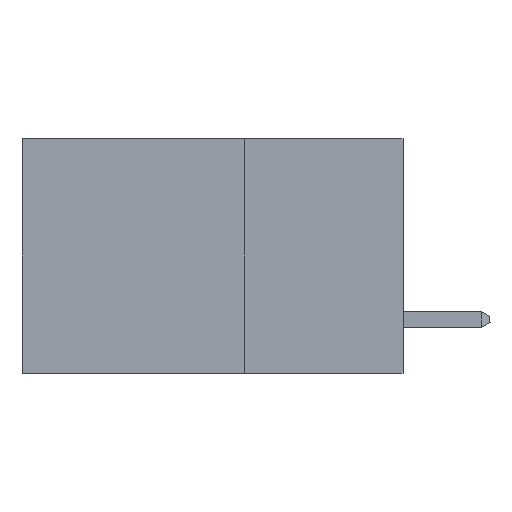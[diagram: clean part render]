
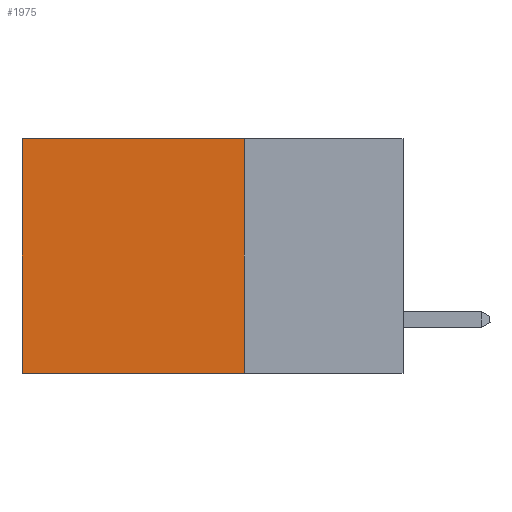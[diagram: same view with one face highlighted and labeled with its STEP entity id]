
A CAD part, left-side view. The second image highlights one B-rep face of the part: STEP entity #1975.
In plain terms, the highlighted planar face has unit normal (-1, 0, 0).
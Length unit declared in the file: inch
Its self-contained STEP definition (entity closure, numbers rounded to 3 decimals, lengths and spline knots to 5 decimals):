
#53 = FACE_OUTER_BOUND ( 'NONE', #13181, .T. ) ;
#1191 = CARTESIAN_POINT ( 'NONE',  ( 0.2875, 0.25, -0.37 ) ) ;
#1975 = ADVANCED_FACE ( 'NONE', ( #53 ), #24681, .F. ) ;
#2242 = ORIENTED_EDGE ( 'NONE', *, *, #23181, .T. ) ;
#3297 = VERTEX_POINT ( 'NONE', #16353 ) ;
#3943 = EDGE_CURVE ( 'NONE', #3297, #7754, #12428, .T. ) ;
#4114 = CARTESIAN_POINT ( 'NONE',  ( 0.2875, 0.6, 0. ) ) ;
#5300 = VECTOR ( 'NONE', #10237, 39.37008 ) ;
#5511 = DIRECTION ( 'NONE',  ( 0., 1., 0. ) ) ;
#7107 = DIRECTION ( 'NONE',  ( 1., 0., 0. ) ) ;
#7754 = VERTEX_POINT ( 'NONE', #9951 ) ;
#7958 = CARTESIAN_POINT ( 'NONE',  ( 0.2875, 0.6, 0. ) ) ;
#8385 = DIRECTION ( 'NONE',  ( 0., 0., -1. ) ) ;
#8970 = ORIENTED_EDGE ( 'NONE', *, *, #15194, .F. ) ;
#9731 = CARTESIAN_POINT ( 'NONE',  ( 0.2875, 0.6, -0.37 ) ) ;
#9815 = LINE ( 'NONE', #16676, #5300 ) ;
#9951 = CARTESIAN_POINT ( 'NONE',  ( 0.2875, 0.25, -0.37 ) ) ;
#10237 = DIRECTION ( 'NONE',  ( 0., 1., 0. ) ) ;
#12428 = LINE ( 'NONE', #23853, #12786 ) ;
#12786 = VECTOR ( 'NONE', #8385, 39.37008 ) ;
#13181 = EDGE_LOOP ( 'NONE', ( #22997, #8970, #25970, #2242 ) ) ;
#15120 = EDGE_CURVE ( 'NONE', #16158, #26685, #21696, .T. ) ;
#15194 = EDGE_CURVE ( 'NONE', #7754, #26685, #18224, .T. ) ;
#16158 = VERTEX_POINT ( 'NONE', #4114 ) ;
#16353 = CARTESIAN_POINT ( 'NONE',  ( 0.2875, 0.25, 0. ) ) ;
#16676 = CARTESIAN_POINT ( 'NONE',  ( 0.2875, 0.25, 0. ) ) ;
#18224 = LINE ( 'NONE', #1191, #20300 ) ;
#20300 = VECTOR ( 'NONE', #5511, 39.37008 ) ;
#20610 = CARTESIAN_POINT ( 'NONE',  ( 0.2875, 0.25, 0. ) ) ;
#21696 = LINE ( 'NONE', #7958, #28220 ) ;
#21870 = AXIS2_PLACEMENT_3D ( 'NONE', #20610, #7107, #26811 ) ;
#22997 = ORIENTED_EDGE ( 'NONE', *, *, #15120, .T. ) ;
#23181 = EDGE_CURVE ( 'NONE', #3297, #16158, #9815, .T. ) ;
#23853 = CARTESIAN_POINT ( 'NONE',  ( 0.2875, 0.25, 0. ) ) ;
#24681 = PLANE ( 'NONE',  #21870 ) ;
#25551 = DIRECTION ( 'NONE',  ( 0., 0., -1. ) ) ;
#25970 = ORIENTED_EDGE ( 'NONE', *, *, #3943, .F. ) ;
#26685 = VERTEX_POINT ( 'NONE', #9731 ) ;
#26811 = DIRECTION ( 'NONE',  ( 0., 0., -1. ) ) ;
#28220 = VECTOR ( 'NONE', #25551, 39.37008 ) ;
